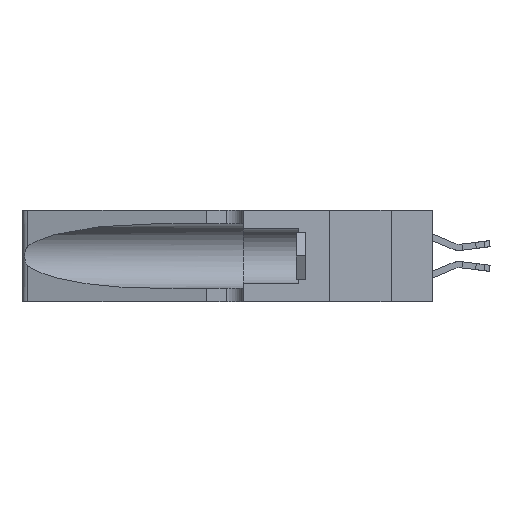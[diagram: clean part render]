
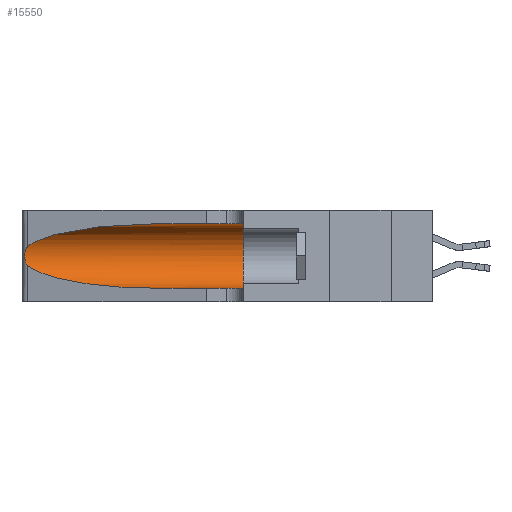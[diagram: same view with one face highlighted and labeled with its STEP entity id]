
A CAD part, left-side view. The second image highlights one B-rep face of the part: STEP entity #15550.
In plain terms, the highlighted cylindrical face has radius 3.308 mm (diameter 6.617 mm), a partial arc.
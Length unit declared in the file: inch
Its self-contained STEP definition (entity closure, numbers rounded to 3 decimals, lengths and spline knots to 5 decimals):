
#559 = CARTESIAN_POINT ( 'NONE',  ( 0.2373, 1.15595, 0.28018 ) ) ;
#597 = CARTESIAN_POINT ( 'NONE',  ( 0.25787, 1.23484, 0.2124 ) ) ;
#603 = B_SPLINE_CURVE_WITH_KNOTS ( 'NONE', 3,
 ( #6694, #9798, #12896, #597, #875, #7039, #11478, #12961, #19275, #6969, #10072, #4000, #2364, #13180 ),
 .UNSPECIFIED., .F., .F.,
 ( 4, 2, 2, 2, 2, 2, 4 ),
 ( 0., 0.00027, 0.00053, 0.00107, 0.0016, 0.00187, 0.00214 ),
 .UNSPECIFIED. ) ;
#875 = CARTESIAN_POINT ( 'NONE',  ( 0.25854, 1.2359, 0.20912 ) ) ;
#888 = EDGE_CURVE ( 'NONE', #17552, #4258, #603, .T. ) ;
#903 = CYLINDRICAL_SURFACE ( 'NONE', #18189, 0.13025 ) ;
#980 = VECTOR ( 'NONE', #5864, 39.37008 ) ;
#1095 = CARTESIAN_POINT ( 'NONE',  ( 0.1305, 1.61858, 0.185 ) ) ;
#1262 = DIRECTION ( 'NONE',  ( 0., 1., 0. ) ) ;
#1492 = EDGE_CURVE ( 'NONE', #7061, #11671, #16192, .T. ) ;
#1799 = AXIS2_PLACEMENT_3D ( 'NONE', #7495, #1262, #7302 ) ;
#2364 = CARTESIAN_POINT ( 'NONE',  ( 0.25555, 1.22993, 0.14849 ) ) ;
#2572 = DIRECTION ( 'NONE',  ( 0., 0., -1. ) ) ;
#4000 = CARTESIAN_POINT ( 'NONE',  ( 0.25639, 1.23186, 0.15144 ) ) ;
#4258 = VERTEX_POINT ( 'NONE', #7075 ) ;
#4789 = CARTESIAN_POINT ( 'NONE',  ( 0.1305, 0.72297, 0.31525 ) ) ;
#5185 = CIRCLE ( 'NONE', #1799, 0.13025 ) ;
#5473 =( BOUNDED_CURVE ( )  B_SPLINE_CURVE ( 3, ( #13146, #12995, #17640, #11449 ),
 .UNSPECIFIED., .F., .F. ) 
 B_SPLINE_CURVE_WITH_KNOTS ( ( 4, 4 ),
 ( 3.44316, 4.71239 ),
 .UNSPECIFIED. ) 
 CURVE ( )  GEOMETRIC_REPRESENTATION_ITEM ( )  RATIONAL_B_SPLINE_CURVE ( ( 1., 0.87, 0.87, 1. ) ) 
 REPRESENTATION_ITEM ( '' )  );
#5864 = DIRECTION ( 'NONE',  ( 0., -1., 0. ) ) ;
#6251 = ORIENTED_EDGE ( 'NONE', *, *, #14550, .T. ) ;
#6605 = EDGE_LOOP ( 'NONE', ( #13020, #9285, #18749, #6251, #18364, #7279 ) ) ;
#6694 = CARTESIAN_POINT ( 'NONE',  ( 0.25487, 1.22718, 0.22369 ) ) ;
#6969 = CARTESIAN_POINT ( 'NONE',  ( 0.25856, 1.23593, 0.16098 ) ) ;
#7039 = CARTESIAN_POINT ( 'NONE',  ( 0.26018, 1.23835, 0.19895 ) ) ;
#7061 = VERTEX_POINT ( 'NONE', #4789 ) ;
#7075 = CARTESIAN_POINT ( 'NONE',  ( 0.25487, 1.22718, 0.14631 ) ) ;
#7279 = ORIENTED_EDGE ( 'NONE', *, *, #1492, .F. ) ;
#7302 = DIRECTION ( 'NONE',  ( 0., 0., 1. ) ) ;
#7407 = VERTEX_POINT ( 'NONE', #12987 ) ;
#7495 = CARTESIAN_POINT ( 'NONE',  ( 0.1305, 0.35, 0.185 ) ) ;
#8776 = CARTESIAN_POINT ( 'NONE',  ( 0.1305, 1.61858, 0.31525 ) ) ;
#9285 = ORIENTED_EDGE ( 'NONE', *, *, #888, .T. ) ;
#9433 = CARTESIAN_POINT ( 'NONE',  ( 0.1305, 0.35, 0.31525 ) ) ;
#9459 = CARTESIAN_POINT ( 'NONE',  ( 0.25487, 1.22718, 0.22369 ) ) ;
#9580 = VERTEX_POINT ( 'NONE', #15219 ) ;
#9798 = CARTESIAN_POINT ( 'NONE',  ( 0.25555, 1.22994, 0.2215 ) ) ;
#10072 = CARTESIAN_POINT ( 'NONE',  ( 0.25789, 1.23486, 0.15765 ) ) ;
#11449 = CARTESIAN_POINT ( 'NONE',  ( 0.1305, 0.72297, 0.05475 ) ) ;
#11478 = CARTESIAN_POINT ( 'NONE',  ( 0.26075, 1.23896, 0.19203 ) ) ;
#11671 = VERTEX_POINT ( 'NONE', #9433 ) ;
#11871 = EDGE_CURVE ( 'NONE', #4258, #9580, #5473, .T. ) ;
#11956 = VECTOR ( 'NONE', #13436, 39.37008 ) ;
#12896 = CARTESIAN_POINT ( 'NONE',  ( 0.25639, 1.23184, 0.21858 ) ) ;
#12961 = CARTESIAN_POINT ( 'NONE',  ( 0.26075, 1.23896, 0.178 ) ) ;
#12987 = CARTESIAN_POINT ( 'NONE',  ( 0.1305, 0.35, 0.05475 ) ) ;
#12995 = CARTESIAN_POINT ( 'NONE',  ( 0.2373, 1.15595, 0.08982 ) ) ;
#13020 = ORIENTED_EDGE ( 'NONE', *, *, #19882, .T. ) ;
#13146 = CARTESIAN_POINT ( 'NONE',  ( 0.25487, 1.22718, 0.14631 ) ) ;
#13180 = CARTESIAN_POINT ( 'NONE',  ( 0.25487, 1.22718, 0.14631 ) ) ;
#13239 = FACE_OUTER_BOUND ( 'NONE', #6605, .T. ) ;
#13409 = DIRECTION ( 'NONE',  ( 0., -1., 0. ) ) ;
#13436 = DIRECTION ( 'NONE',  ( 0., -1., 0. ) ) ;
#14349 = CARTESIAN_POINT ( 'NONE',  ( 0.25487, 1.22718, 0.22369 ) ) ;
#14550 = EDGE_CURVE ( 'NONE', #9580, #7407, #18898, .T. ) ;
#15219 = CARTESIAN_POINT ( 'NONE',  ( 0.1305, 0.72297, 0.05475 ) ) ;
#15550 = ADVANCED_FACE ( 'NONE', ( #13239 ), #903, .F. ) ;
#16192 = LINE ( 'NONE', #8776, #980 ) ;
#17552 = VERTEX_POINT ( 'NONE', #9459 ) ;
#17640 = CARTESIAN_POINT ( 'NONE',  ( 0.18966, 0.96281, 0.05475 ) ) ;
#17839 = EDGE_CURVE ( 'NONE', #11671, #7407, #5185, .T. ) ;
#18048 = CARTESIAN_POINT ( 'NONE',  ( 0.1305, 1.61858, 0.05475 ) ) ;
#18189 = AXIS2_PLACEMENT_3D ( 'NONE', #1095, #13409, #2572 ) ;
#18364 = ORIENTED_EDGE ( 'NONE', *, *, #17839, .F. ) ;
#18749 = ORIENTED_EDGE ( 'NONE', *, *, #11871, .T. ) ;
#18898 = LINE ( 'NONE', #18048, #11956 ) ;
#19161 = CARTESIAN_POINT ( 'NONE',  ( 0.1305, 0.72297, 0.31525 ) ) ;
#19226 = CARTESIAN_POINT ( 'NONE',  ( 0.18966, 0.96281, 0.31525 ) ) ;
#19275 = CARTESIAN_POINT ( 'NONE',  ( 0.26017, 1.23833, 0.17102 ) ) ;
#19527 =( BOUNDED_CURVE ( )  B_SPLINE_CURVE ( 3, ( #19161, #19226, #559, #14349 ),
 .UNSPECIFIED., .F., .F. ) 
 B_SPLINE_CURVE_WITH_KNOTS ( ( 4, 4 ),
 ( 1.5708, 2.84003 ),
 .UNSPECIFIED. ) 
 CURVE ( )  GEOMETRIC_REPRESENTATION_ITEM ( )  RATIONAL_B_SPLINE_CURVE ( ( 1., 0.87, 0.87, 1. ) ) 
 REPRESENTATION_ITEM ( '' )  );
#19882 = EDGE_CURVE ( 'NONE', #7061, #17552, #19527, .T. ) ;
